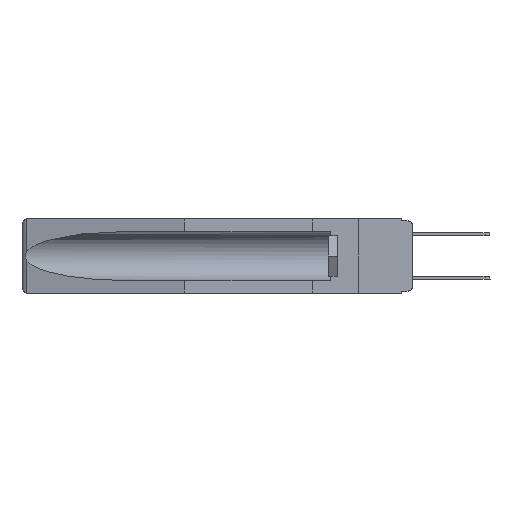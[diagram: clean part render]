
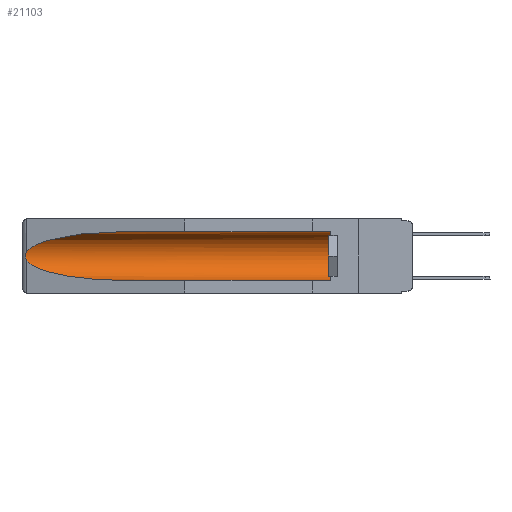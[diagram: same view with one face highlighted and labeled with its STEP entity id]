
A CAD part, left-side view. The second image highlights one B-rep face of the part: STEP entity #21103.
In plain terms, the highlighted cylindrical face has radius 2.857 mm (diameter 5.715 mm), a partial arc.
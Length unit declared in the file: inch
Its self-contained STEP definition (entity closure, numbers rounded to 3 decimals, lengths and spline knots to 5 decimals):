
#133 = EDGE_CURVE ( 'NONE', #5751, #9531, #19349, .T. ) ;
#446 = CYLINDRICAL_SURFACE ( 'NONE', #8718, 0.1125 ) ;
#631 = CARTESIAN_POINT ( 'NONE',  ( 0.26597, 1.5296, -0.19026 ) ) ;
#712 = EDGE_CURVE ( 'NONE', #5751, #10858, #982, .T. ) ;
#982 = LINE ( 'NONE', #5789, #14163 ) ;
#1520 =( BOUNDED_CURVE ( )  B_SPLINE_CURVE ( 3, ( #4118, #9733, #5963, #13252 ),
 .UNSPECIFIED., .F., .F. ) 
 B_SPLINE_CURVE_WITH_KNOTS ( ( 4, 4 ),
 ( 4.71239, 6.08839 ),
 .UNSPECIFIED. ) 
 CURVE ( )  GEOMETRIC_REPRESENTATION_ITEM ( )  RATIONAL_B_SPLINE_CURVE ( ( 1., 0.848, 0.848, 1. ) ) 
 REPRESENTATION_ITEM ( '' )  );
#3389 = CARTESIAN_POINT ( 'NONE',  ( 0.155, 1.07973, -0.284 ) ) ;
#4000 = EDGE_LOOP ( 'NONE', ( #14036, #12027, #9418, #11898, #7733, #18097 ) ) ;
#4118 = CARTESIAN_POINT ( 'NONE',  ( 0.155, 1.07973, -0.059 ) ) ;
#4785 = CARTESIAN_POINT ( 'NONE',  ( 0.26537, 1.52718, -0.19328 ) ) ;
#5472 = CARTESIAN_POINT ( 'NONE',  ( 0.155, 0.126, -0.1715 ) ) ;
#5751 = VERTEX_POINT ( 'NONE', #21939 ) ;
#5789 = CARTESIAN_POINT ( 'NONE',  ( 0.155, -0.30754, -0.284 ) ) ;
#5963 = CARTESIAN_POINT ( 'NONE',  ( 0.25451, 1.48313, -0.09465 ) ) ;
#6237 = CARTESIAN_POINT ( 'NONE',  ( 0.2675, 1.53308, -0.16763 ) ) ;
#7614 = DIRECTION ( 'NONE',  ( 0., -1., 0. ) ) ;
#7733 = ORIENTED_EDGE ( 'NONE', *, *, #133, .T. ) ;
#8427 = EDGE_CURVE ( 'NONE', #9531, #19263, #19184, .T. ) ;
#8718 = AXIS2_PLACEMENT_3D ( 'NONE', #11549, #20568, #13302 ) ;
#9418 = ORIENTED_EDGE ( 'NONE', *, *, #20893, .T. ) ;
#9451 = CARTESIAN_POINT ( 'NONE',  ( 0.26537, 1.52718, -0.14972 ) ) ;
#9531 = VERTEX_POINT ( 'NONE', #16027 ) ;
#9733 = CARTESIAN_POINT ( 'NONE',  ( 0.21114, 1.30732, -0.059 ) ) ;
#9741 = CARTESIAN_POINT ( 'NONE',  ( 0.155, 1.07973, -0.059 ) ) ;
#10071 = CARTESIAN_POINT ( 'NONE',  ( 0.26537, 1.52718, -0.19328 ) ) ;
#10465 = FACE_OUTER_BOUND ( 'NONE', #4000, .T. ) ;
#10858 = VERTEX_POINT ( 'NONE', #3389 ) ;
#11481 = DIRECTION ( 'NONE',  ( 0., 1., 0. ) ) ;
#11522 = CARTESIAN_POINT ( 'NONE',  ( 0.26597, 1.52961, -0.15275 ) ) ;
#11549 = CARTESIAN_POINT ( 'NONE',  ( 0.155, -0.30754, -0.1715 ) ) ;
#11751 = CARTESIAN_POINT ( 'NONE',  ( 0.2673, 1.53269, -0.17917 ) ) ;
#11898 = ORIENTED_EDGE ( 'NONE', *, *, #712, .F. ) ;
#12027 = ORIENTED_EDGE ( 'NONE', *, *, #16861, .T. ) ;
#12691 = CARTESIAN_POINT ( 'NONE',  ( 0.21114, 1.30732, -0.284 ) ) ;
#13252 = CARTESIAN_POINT ( 'NONE',  ( 0.26537, 1.52718, -0.14972 ) ) ;
#13302 = DIRECTION ( 'NONE',  ( 0., 0., 1. ) ) ;
#13598 = CARTESIAN_POINT ( 'NONE',  ( 0.2675, 1.53308, -0.17534 ) ) ;
#14036 = ORIENTED_EDGE ( 'NONE', *, *, #17461, .T. ) ;
#14163 = VECTOR ( 'NONE', #11481, 39.37008 ) ;
#14509 = CARTESIAN_POINT ( 'NONE',  ( 0.155, 1.07973, -0.284 ) ) ;
#14681 = DIRECTION ( 'NONE',  ( 0., 1., 0. ) ) ;
#14724 = VERTEX_POINT ( 'NONE', #4785 ) ;
#14889 = DIRECTION ( 'NONE',  ( 0., 0., 1. ) ) ;
#16027 = CARTESIAN_POINT ( 'NONE',  ( 0.155, 0.126, -0.059 ) ) ;
#16433 = VECTOR ( 'NONE', #14681, 39.37008 ) ;
#16861 = EDGE_CURVE ( 'NONE', #18381, #14724, #17492, .T. ) ;
#17191 = CARTESIAN_POINT ( 'NONE',  ( 0.2673, 1.5327, -0.16383 ) ) ;
#17461 = EDGE_CURVE ( 'NONE', #19263, #18381, #1520, .T. ) ;
#17492 = B_SPLINE_CURVE_WITH_KNOTS ( 'NONE', 3,
 ( #9451, #11522, #22863, #17191, #6237, #13598, #11751, #18970, #631, #10071 ),
 .UNSPECIFIED., .F., .F.,
 ( 4, 2, 2, 2, 4 ),
 ( 0., 0.00029, 0.00058, 0.00087, 0.00117 ),
 .UNSPECIFIED. ) ;
#17719 = AXIS2_PLACEMENT_3D ( 'NONE', #5472, #7614, #14889 ) ;
#17999 = CARTESIAN_POINT ( 'NONE',  ( 0.26537, 1.52718, -0.14972 ) ) ;
#18097 = ORIENTED_EDGE ( 'NONE', *, *, #8427, .T. ) ;
#18120 = CARTESIAN_POINT ( 'NONE',  ( 0.26537, 1.52718, -0.19328 ) ) ;
#18381 = VERTEX_POINT ( 'NONE', #17999 ) ;
#18970 = CARTESIAN_POINT ( 'NONE',  ( 0.26655, 1.53094, -0.18657 ) ) ;
#19184 = LINE ( 'NONE', #22030, #16433 ) ;
#19263 = VERTEX_POINT ( 'NONE', #9741 ) ;
#19349 = CIRCLE ( 'NONE', #17719, 0.1125 ) ;
#20568 = DIRECTION ( 'NONE',  ( 0., 1., 0. ) ) ;
#20893 = EDGE_CURVE ( 'NONE', #14724, #10858, #23084, .T. ) ;
#21103 = ADVANCED_FACE ( 'NONE', ( #10465 ), #446, .F. ) ;
#21939 = CARTESIAN_POINT ( 'NONE',  ( 0.155, 0.126, -0.284 ) ) ;
#22030 = CARTESIAN_POINT ( 'NONE',  ( 0.155, -0.30754, -0.059 ) ) ;
#22863 = CARTESIAN_POINT ( 'NONE',  ( 0.26654, 1.53092, -0.15636 ) ) ;
#23084 =( BOUNDED_CURVE ( )  B_SPLINE_CURVE ( 3, ( #18120, #23641, #12691, #14509 ),
 .UNSPECIFIED., .F., .F. ) 
 B_SPLINE_CURVE_WITH_KNOTS ( ( 4, 4 ),
 ( 0.1948, 1.5708 ),
 .UNSPECIFIED. ) 
 CURVE ( )  GEOMETRIC_REPRESENTATION_ITEM ( )  RATIONAL_B_SPLINE_CURVE ( ( 1., 0.848, 0.848, 1. ) ) 
 REPRESENTATION_ITEM ( '' )  );
#23641 = CARTESIAN_POINT ( 'NONE',  ( 0.25451, 1.48313, -0.24835 ) ) ;
